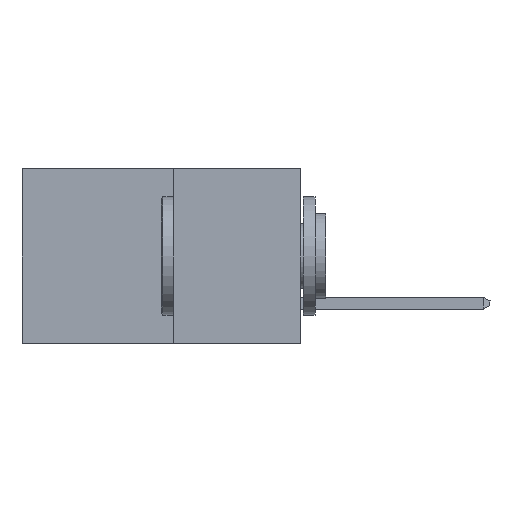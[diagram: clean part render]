
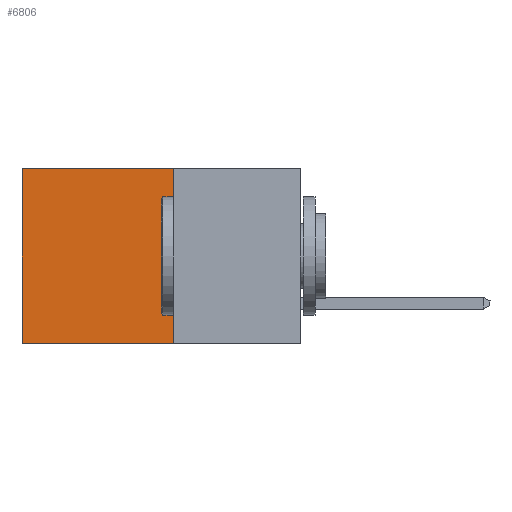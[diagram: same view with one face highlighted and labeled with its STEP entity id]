
A CAD part, left-side view. The second image highlights one B-rep face of the part: STEP entity #6806.
In plain terms, the highlighted planar face has unit normal (-1, 0, 0).
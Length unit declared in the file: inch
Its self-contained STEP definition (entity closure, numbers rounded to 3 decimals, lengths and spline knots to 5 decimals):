
#1 = PLANE ( 'NONE',  #9266 ) ;
#24 = CARTESIAN_POINT ( 'NONE',  ( 0.277, 0.27, -0.37 ) ) ;
#395 = CARTESIAN_POINT ( 'NONE',  ( 0.277, 0.27, -0.37 ) ) ;
#439 = CARTESIAN_POINT ( 'NONE',  ( 0.277, 0.59, 0. ) ) ;
#657 = EDGE_CURVE ( 'NONE', #8104, #4618, #2765, .T. ) ;
#737 = LINE ( 'NONE', #6082, #4508 ) ;
#779 = VECTOR ( 'NONE', #1970, 39.37008 ) ;
#1965 = CARTESIAN_POINT ( 'NONE',  ( 0.277, 0.59, -0.37 ) ) ;
#1970 = DIRECTION ( 'NONE',  ( 0., 0., -1. ) ) ;
#2371 = ORIENTED_EDGE ( 'NONE', *, *, #9122, .T. ) ;
#2412 = EDGE_CURVE ( 'NONE', #4618, #3882, #737, .T. ) ;
#2448 = ORIENTED_EDGE ( 'NONE', *, *, #2412, .F. ) ;
#2765 = LINE ( 'NONE', #3691, #779 ) ;
#2955 = CARTESIAN_POINT ( 'NONE',  ( 0.277, 0.59, -0.37 ) ) ;
#3051 = EDGE_LOOP ( 'NONE', ( #2371, #2448, #6578, #7284 ) ) ;
#3531 = VERTEX_POINT ( 'NONE', #439 ) ;
#3691 = CARTESIAN_POINT ( 'NONE',  ( 0.277, 0.27, -0.37 ) ) ;
#3865 = LINE ( 'NONE', #8022, #5561 ) ;
#3882 = VERTEX_POINT ( 'NONE', #1965 ) ;
#4255 = FACE_OUTER_BOUND ( 'NONE', #3051, .T. ) ;
#4508 = VECTOR ( 'NONE', #6071, 39.37008 ) ;
#4618 = VERTEX_POINT ( 'NONE', #395 ) ;
#5561 = VECTOR ( 'NONE', #7314, 39.37008 ) ;
#6071 = DIRECTION ( 'NONE',  ( 0., 1., 0. ) ) ;
#6082 = CARTESIAN_POINT ( 'NONE',  ( 0.277, 0.27, -0.37 ) ) ;
#6327 = VECTOR ( 'NONE', #7980, 39.37008 ) ;
#6333 = CARTESIAN_POINT ( 'NONE',  ( 0.277, 0.27, 0. ) ) ;
#6578 = ORIENTED_EDGE ( 'NONE', *, *, #657, .F. ) ;
#6806 = ADVANCED_FACE ( 'NONE', ( #4255 ), #1, .F. ) ;
#7284 = ORIENTED_EDGE ( 'NONE', *, *, #8454, .T. ) ;
#7314 = DIRECTION ( 'NONE',  ( 0., 1., 0. ) ) ;
#7980 = DIRECTION ( 'NONE',  ( 0., 0., -1. ) ) ;
#8022 = CARTESIAN_POINT ( 'NONE',  ( 0.277, 0.27, 0. ) ) ;
#8104 = VERTEX_POINT ( 'NONE', #6333 ) ;
#8388 = LINE ( 'NONE', #2955, #6327 ) ;
#8454 = EDGE_CURVE ( 'NONE', #8104, #3531, #3865, .T. ) ;
#8772 = DIRECTION ( 'NONE',  ( 1., 0., 0. ) ) ;
#8860 = DIRECTION ( 'NONE',  ( 0., 0., -1. ) ) ;
#9122 = EDGE_CURVE ( 'NONE', #3531, #3882, #8388, .T. ) ;
#9266 = AXIS2_PLACEMENT_3D ( 'NONE', #24, #8772, #8860 ) ;
